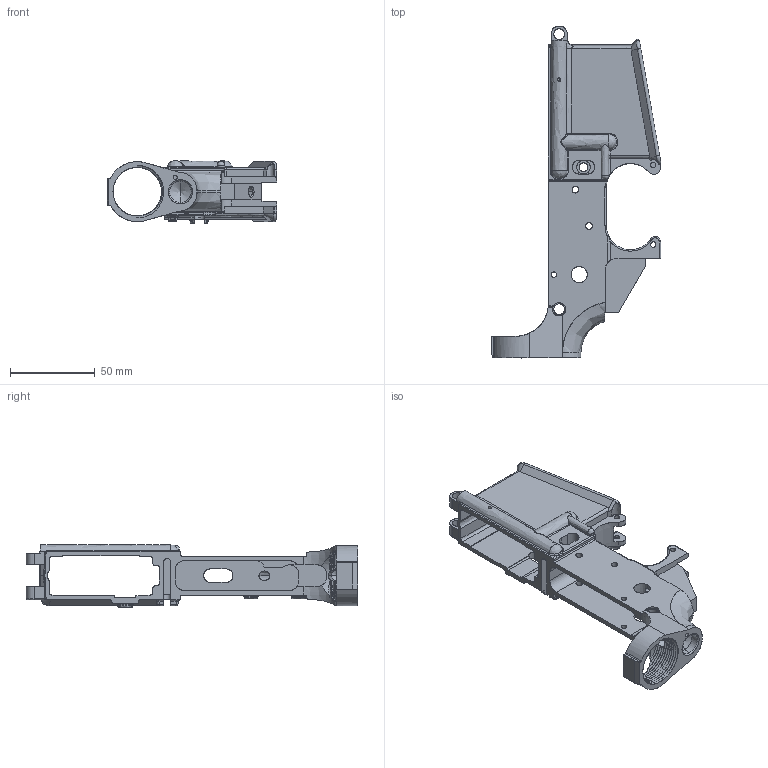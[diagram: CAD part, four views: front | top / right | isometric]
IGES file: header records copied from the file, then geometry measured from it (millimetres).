
Start section: XXXXXXXXXXXXXXXXXXXXXXXXXXXXXXXXXXXXXXXXXXXXXXXXXXXXXXXXXXXXXXX
Global section: file name: XXXXXXXXXXXXXXXXXXXXXXXXXXXXXXXXXXXXXXXXXXXXXXXXXXXXXXX; native system: XXXXXXXXXXXXXXX; preprocessor: XXXXXXXXXXXXXXX; author: XXXXXXXXXXXXXXX; date: 110829.153408; units: inch
Bounding box: 99.8 x 195.35 x 36.83 mm (x, y, z)
Surface area: 53002.6 mm2 (no closed solid volume)
Topology: 0 solids, 0 shells, 519 faces, 8669 edges, 8653 vertices
Faces by surface type: revolution 260, bspline 259
